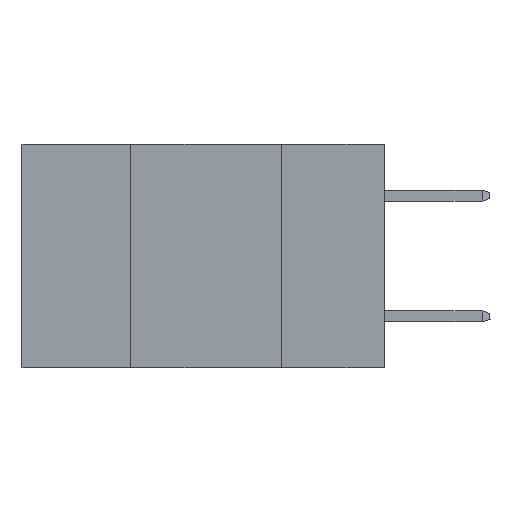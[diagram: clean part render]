
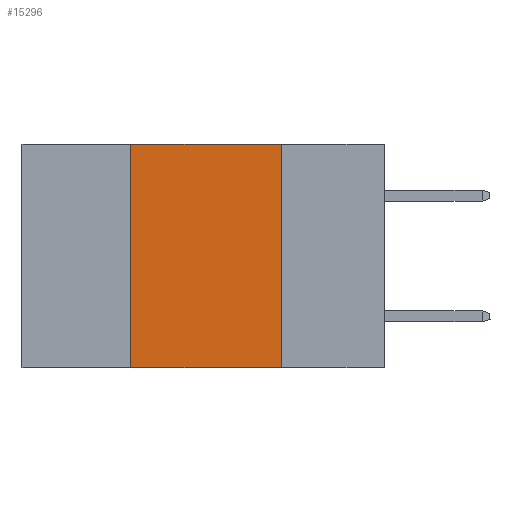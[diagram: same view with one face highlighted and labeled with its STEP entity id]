
A CAD part, left-side view. The second image highlights one B-rep face of the part: STEP entity #15296.
In plain terms, the highlighted planar face has unit normal (-1, 0, 0).
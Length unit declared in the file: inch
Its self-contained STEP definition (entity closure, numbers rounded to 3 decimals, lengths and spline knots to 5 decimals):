
#387 = DIRECTION ( 'NONE',  ( 0., -1., 0. ) ) ;
#688 = ORIENTED_EDGE ( 'NONE', *, *, #14346, .F. ) ;
#1322 = CARTESIAN_POINT ( 'NONE',  ( 0., 0.6, 0. ) ) ;
#1881 = DIRECTION ( 'NONE',  ( 0., 0., 1. ) ) ;
#2086 = VECTOR ( 'NONE', #387, 39.37008 ) ;
#2926 = LINE ( 'NONE', #14527, #10822 ) ;
#3016 = DIRECTION ( 'NONE',  ( 1., 0., 0. ) ) ;
#4022 = VERTEX_POINT ( 'NONE', #19512 ) ;
#5765 = CARTESIAN_POINT ( 'NONE',  ( 0., 0.17, 0. ) ) ;
#6271 = VERTEX_POINT ( 'NONE', #7070 ) ;
#6638 = CARTESIAN_POINT ( 'NONE',  ( 0., 0.17, -0.37 ) ) ;
#6812 = CARTESIAN_POINT ( 'NONE',  ( 0., 0.42, -0.37 ) ) ;
#6942 = LINE ( 'NONE', #19099, #2086 ) ;
#7070 = CARTESIAN_POINT ( 'NONE',  ( 0., 0.42, 0. ) ) ;
#7143 = ORIENTED_EDGE ( 'NONE', *, *, #12332, .T. ) ;
#7516 = VECTOR ( 'NONE', #16447, 39.37008 ) ;
#7562 = VERTEX_POINT ( 'NONE', #6638 ) ;
#8241 = EDGE_LOOP ( 'NONE', ( #12355, #688, #10713, #7143 ) ) ;
#10713 = ORIENTED_EDGE ( 'NONE', *, *, #12937, .F. ) ;
#10822 = VECTOR ( 'NONE', #16053, 39.37008 ) ;
#10878 = PLANE ( 'NONE',  #12929 ) ;
#11875 = VERTEX_POINT ( 'NONE', #5765 ) ;
#12332 = EDGE_CURVE ( 'NONE', #4022, #7562, #2926, .T. ) ;
#12355 = ORIENTED_EDGE ( 'NONE', *, *, #19161, .F. ) ;
#12929 = AXIS2_PLACEMENT_3D ( 'NONE', #1322, #3016, #13893 ) ;
#12937 = EDGE_CURVE ( 'NONE', #4022, #6271, #15985, .T. ) ;
#13534 = FACE_OUTER_BOUND ( 'NONE', #8241, .T. ) ;
#13893 = DIRECTION ( 'NONE',  ( 0., 0., -1. ) ) ;
#14346 = EDGE_CURVE ( 'NONE', #6271, #11875, #6942, .T. ) ;
#14527 = CARTESIAN_POINT ( 'NONE',  ( 0., 0.6, -0.37 ) ) ;
#14903 = CARTESIAN_POINT ( 'NONE',  ( 0., 0.17, -0.37 ) ) ;
#15296 = ADVANCED_FACE ( 'NONE', ( #13534 ), #10878, .F. ) ;
#15985 = LINE ( 'NONE', #6812, #18616 ) ;
#16053 = DIRECTION ( 'NONE',  ( 0., -1., 0. ) ) ;
#16447 = DIRECTION ( 'NONE',  ( 0., 0., -1. ) ) ;
#18616 = VECTOR ( 'NONE', #1881, 39.37008 ) ;
#19099 = CARTESIAN_POINT ( 'NONE',  ( 0., 0.6, 0. ) ) ;
#19161 = EDGE_CURVE ( 'NONE', #11875, #7562, #19583, .T. ) ;
#19512 = CARTESIAN_POINT ( 'NONE',  ( 0., 0.42, -0.37 ) ) ;
#19583 = LINE ( 'NONE', #14903, #7516 ) ;
